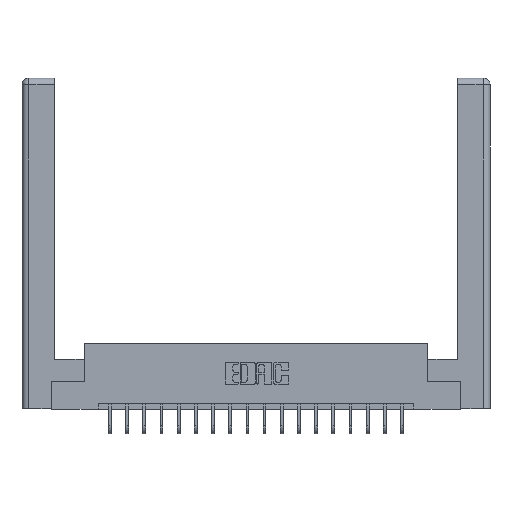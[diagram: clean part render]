
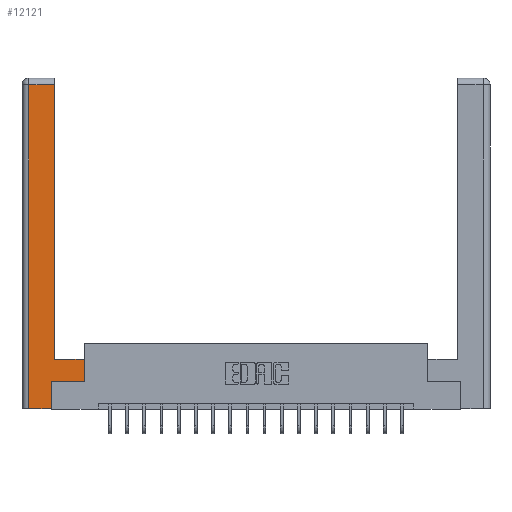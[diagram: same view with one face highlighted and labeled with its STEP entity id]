
A CAD part, top view. The second image highlights one B-rep face of the part: STEP entity #12121.
In plain terms, the highlighted planar face has unit normal (0, 0, 1).
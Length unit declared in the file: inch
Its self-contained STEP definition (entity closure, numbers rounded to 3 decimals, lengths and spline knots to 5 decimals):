
#43 = DIRECTION ( 'NONE',  ( -1., 0., 0. ) ) ;
#841 = EDGE_CURVE ( 'NONE', #6522, #2586, #990, .T. ) ;
#876 = ORIENTED_EDGE ( 'NONE', *, *, #12939, .T. ) ;
#990 = LINE ( 'NONE', #18574, #8792 ) ;
#1710 = CARTESIAN_POINT ( 'NONE',  ( 0.265, 0., 0. ) ) ;
#1775 = LINE ( 'NONE', #10972, #10947 ) ;
#1983 = DIRECTION ( 'NONE',  ( 0., 0., -1. ) ) ;
#1988 = CARTESIAN_POINT ( 'NONE',  ( 0.565, 0.45, 0. ) ) ;
#2004 = VECTOR ( 'NONE', #43, 39.37008 ) ;
#2531 = ORIENTED_EDGE ( 'NONE', *, *, #841, .T. ) ;
#2586 = VERTEX_POINT ( 'NONE', #15123 ) ;
#2822 = CARTESIAN_POINT ( 'NONE',  ( 0.265, 0.245, 0. ) ) ;
#3007 = VERTEX_POINT ( 'NONE', #10891 ) ;
#3166 = LINE ( 'NONE', #19345, #14842 ) ;
#3327 = VECTOR ( 'NONE', #20937, 39.37008 ) ;
#3566 = ORIENTED_EDGE ( 'NONE', *, *, #16064, .T. ) ;
#5416 = EDGE_CURVE ( 'NONE', #2586, #14308, #13812, .T. ) ;
#6125 = DIRECTION ( 'NONE',  ( 0., 1., 0. ) ) ;
#6286 = CARTESIAN_POINT ( 'NONE',  ( 0.265, 0., 0. ) ) ;
#6362 = EDGE_CURVE ( 'NONE', #14308, #9013, #14522, .T. ) ;
#6522 = VERTEX_POINT ( 'NONE', #10830 ) ;
#7045 = EDGE_CURVE ( 'NONE', #13460, #12907, #14258, .T. ) ;
#7717 = CARTESIAN_POINT ( 'NONE',  ( 0.0615, 2.94, 0. ) ) ;
#8525 = LINE ( 'NONE', #11515, #2004 ) ;
#8792 = VECTOR ( 'NONE', #19946, 39.37008 ) ;
#9013 = VERTEX_POINT ( 'NONE', #19893 ) ;
#9071 = VECTOR ( 'NONE', #10610, 39.37008 ) ;
#9159 = CARTESIAN_POINT ( 'NONE',  ( 0.565, 0.45, 0. ) ) ;
#9398 = VECTOR ( 'NONE', #9605, 39.37008 ) ;
#9605 = DIRECTION ( 'NONE',  ( 1., 0., 0. ) ) ;
#9860 = VECTOR ( 'NONE', #13015, 39.37008 ) ;
#10229 = CARTESIAN_POINT ( 'NONE',  ( 0., 0., 0. ) ) ;
#10610 = DIRECTION ( 'NONE',  ( 0., 1., 0. ) ) ;
#10715 = VERTEX_POINT ( 'NONE', #20392 ) ;
#10830 = CARTESIAN_POINT ( 'NONE',  ( 0.0615, 2.94, 0. ) ) ;
#10891 = CARTESIAN_POINT ( 'NONE',  ( 0.295, 2.94, 0. ) ) ;
#10947 = VECTOR ( 'NONE', #16073, 39.37008 ) ;
#10972 = CARTESIAN_POINT ( 'NONE',  ( 0.565, 0.245, 0. ) ) ;
#11515 = CARTESIAN_POINT ( 'NONE',  ( 0.295, 0.45, 0. ) ) ;
#11922 = LINE ( 'NONE', #7717, #3327 ) ;
#11945 = EDGE_LOOP ( 'NONE', ( #876, #3566, #2531, #13425, #20395, #13097, #17739, #14253 ) ) ;
#12121 = ADVANCED_FACE ( 'NONE', ( #19285 ), #16989, .F. ) ;
#12907 = VERTEX_POINT ( 'NONE', #9159 ) ;
#12939 = EDGE_CURVE ( 'NONE', #10715, #3007, #3166, .T. ) ;
#13015 = DIRECTION ( 'NONE',  ( 0., 1., 0. ) ) ;
#13097 = ORIENTED_EDGE ( 'NONE', *, *, #15097, .T. ) ;
#13425 = ORIENTED_EDGE ( 'NONE', *, *, #5416, .T. ) ;
#13460 = VERTEX_POINT ( 'NONE', #16316 ) ;
#13634 = DIRECTION ( 'NONE',  ( -1., 0., 0. ) ) ;
#13812 = LINE ( 'NONE', #6286, #9398 ) ;
#14253 = ORIENTED_EDGE ( 'NONE', *, *, #15586, .T. ) ;
#14258 = LINE ( 'NONE', #1988, #9071 ) ;
#14308 = VERTEX_POINT ( 'NONE', #1710 ) ;
#14522 = LINE ( 'NONE', #2822, #9860 ) ;
#14842 = VECTOR ( 'NONE', #6125, 39.37008 ) ;
#15097 = EDGE_CURVE ( 'NONE', #9013, #13460, #1775, .T. ) ;
#15123 = CARTESIAN_POINT ( 'NONE',  ( 0.0615, 0., 0. ) ) ;
#15586 = EDGE_CURVE ( 'NONE', #12907, #10715, #8525, .T. ) ;
#16064 = EDGE_CURVE ( 'NONE', #3007, #6522, #11922, .T. ) ;
#16073 = DIRECTION ( 'NONE',  ( 1., 0., 0. ) ) ;
#16316 = CARTESIAN_POINT ( 'NONE',  ( 0.565, 0.245, 0. ) ) ;
#16989 = PLANE ( 'NONE',  #18784 ) ;
#17739 = ORIENTED_EDGE ( 'NONE', *, *, #7045, .T. ) ;
#18574 = CARTESIAN_POINT ( 'NONE',  ( 0.0615, 0., 0. ) ) ;
#18784 = AXIS2_PLACEMENT_3D ( 'NONE', #10229, #1983, #13634 ) ;
#19285 = FACE_OUTER_BOUND ( 'NONE', #11945, .T. ) ;
#19345 = CARTESIAN_POINT ( 'NONE',  ( 0.295, 3., 0. ) ) ;
#19893 = CARTESIAN_POINT ( 'NONE',  ( 0.265, 0.245, 0. ) ) ;
#19946 = DIRECTION ( 'NONE',  ( 0., -1., 0. ) ) ;
#20392 = CARTESIAN_POINT ( 'NONE',  ( 0.295, 0.45, 0. ) ) ;
#20395 = ORIENTED_EDGE ( 'NONE', *, *, #6362, .T. ) ;
#20937 = DIRECTION ( 'NONE',  ( -1., 0., 0. ) ) ;
